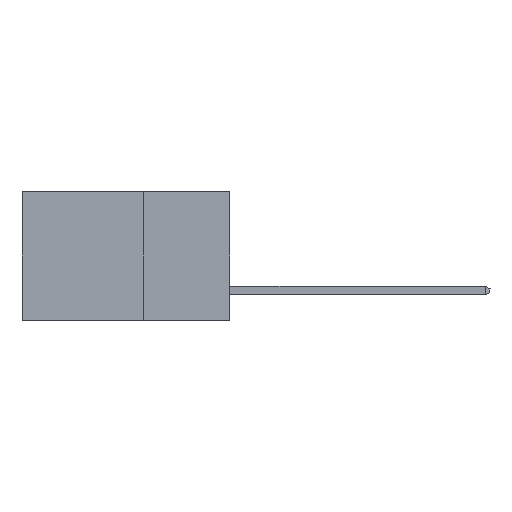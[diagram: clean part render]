
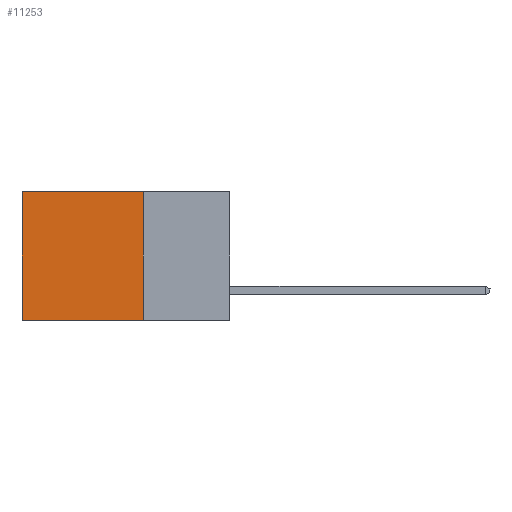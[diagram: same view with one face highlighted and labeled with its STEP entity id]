
A CAD part, left-side view. The second image highlights one B-rep face of the part: STEP entity #11253.
In plain terms, the highlighted planar face has unit normal (-1, 0, 0).
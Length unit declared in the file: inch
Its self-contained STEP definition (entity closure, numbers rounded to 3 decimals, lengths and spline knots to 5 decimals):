
#997 = CARTESIAN_POINT ( 'NONE',  ( 0.298, 0.25, -0.37 ) ) ;
#1636 = CARTESIAN_POINT ( 'NONE',  ( 0.298, 0.25, -0.37 ) ) ;
#2499 = AXIS2_PLACEMENT_3D ( 'NONE', #3946, #13615, #13519 ) ;
#2624 = PLANE ( 'NONE',  #2499 ) ;
#2634 = CARTESIAN_POINT ( 'NONE',  ( 0.298, 0.25, 0. ) ) ;
#3284 = EDGE_CURVE ( 'NONE', #9943, #10635, #14778, .T. ) ;
#3330 = CARTESIAN_POINT ( 'NONE',  ( 0.298, 0.6, -0.37 ) ) ;
#3946 = CARTESIAN_POINT ( 'NONE',  ( 0.298, 0.25, 0. ) ) ;
#4183 = CARTESIAN_POINT ( 'NONE',  ( 0.298, 0.25, 0. ) ) ;
#4229 = EDGE_CURVE ( 'NONE', #6026, #10635, #10351, .T. ) ;
#4771 = EDGE_CURVE ( 'NONE', #14367, #9943, #8283, .T. ) ;
#5237 = DIRECTION ( 'NONE',  ( 0., 0., -1. ) ) ;
#5280 = DIRECTION ( 'NONE',  ( 0., 1., 0. ) ) ;
#6026 = VERTEX_POINT ( 'NONE', #997 ) ;
#6487 = EDGE_CURVE ( 'NONE', #14367, #6026, #11066, .T. ) ;
#6577 = EDGE_LOOP ( 'NONE', ( #11674, #13875, #13206, #12676 ) ) ;
#6688 = DIRECTION ( 'NONE',  ( 0., 0., -1. ) ) ;
#7588 = FACE_OUTER_BOUND ( 'NONE', #6577, .T. ) ;
#7750 = CARTESIAN_POINT ( 'NONE',  ( 0.298, 0.6, 0. ) ) ;
#8283 = LINE ( 'NONE', #13940, #15445 ) ;
#9104 = DIRECTION ( 'NONE',  ( 0., 1., 0. ) ) ;
#9943 = VERTEX_POINT ( 'NONE', #14072 ) ;
#10351 = LINE ( 'NONE', #1636, #14149 ) ;
#10635 = VERTEX_POINT ( 'NONE', #3330 ) ;
#11066 = LINE ( 'NONE', #4183, #14683 ) ;
#11253 = ADVANCED_FACE ( 'NONE', ( #7588 ), #2624, .F. ) ;
#11674 = ORIENTED_EDGE ( 'NONE', *, *, #3284, .T. ) ;
#11910 = VECTOR ( 'NONE', #6688, 39.37008 ) ;
#12676 = ORIENTED_EDGE ( 'NONE', *, *, #4771, .T. ) ;
#13206 = ORIENTED_EDGE ( 'NONE', *, *, #6487, .F. ) ;
#13519 = DIRECTION ( 'NONE',  ( 0., 0., -1. ) ) ;
#13615 = DIRECTION ( 'NONE',  ( 1., 0., 0. ) ) ;
#13875 = ORIENTED_EDGE ( 'NONE', *, *, #4229, .F. ) ;
#13940 = CARTESIAN_POINT ( 'NONE',  ( 0.298, 0.25, 0. ) ) ;
#14072 = CARTESIAN_POINT ( 'NONE',  ( 0.298, 0.6, 0. ) ) ;
#14149 = VECTOR ( 'NONE', #5280, 39.37008 ) ;
#14367 = VERTEX_POINT ( 'NONE', #2634 ) ;
#14683 = VECTOR ( 'NONE', #5237, 39.37008 ) ;
#14778 = LINE ( 'NONE', #7750, #11910 ) ;
#15445 = VECTOR ( 'NONE', #9104, 39.37008 ) ;
